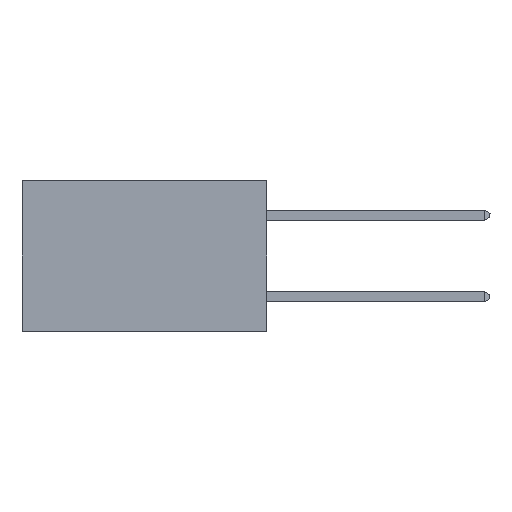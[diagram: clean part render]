
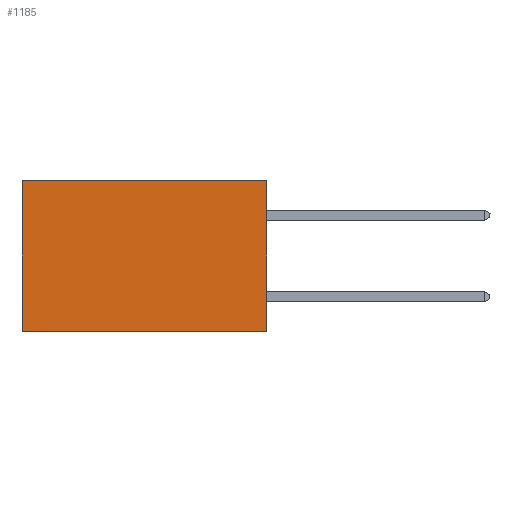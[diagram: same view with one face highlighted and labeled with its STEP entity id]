
A CAD part, left-side view. The second image highlights one B-rep face of the part: STEP entity #1185.
In plain terms, the highlighted planar face has unit normal (-1, 0, 0).
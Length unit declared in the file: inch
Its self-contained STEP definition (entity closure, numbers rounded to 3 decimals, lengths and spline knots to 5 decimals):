
#76 = VECTOR ( 'NONE', #9339, 39.37008 ) ;
#114 = LINE ( 'NONE', #5655, #15353 ) ;
#429 = CARTESIAN_POINT ( 'NONE',  ( 0.2875, 0., 0. ) ) ;
#536 = LINE ( 'NONE', #7866, #76 ) ;
#741 = ORIENTED_EDGE ( 'NONE', *, *, #16037, .F. ) ;
#1185 = ADVANCED_FACE ( 'NONE', ( #12758 ), #17254, .F. ) ;
#1189 = DIRECTION ( 'NONE',  ( 0., 0., -1. ) ) ;
#1426 = EDGE_LOOP ( 'NONE', ( #10645, #2452, #741, #5176 ) ) ;
#1536 = VERTEX_POINT ( 'NONE', #9140 ) ;
#2118 = AXIS2_PLACEMENT_3D ( 'NONE', #15785, #18692, #9932 ) ;
#2452 = ORIENTED_EDGE ( 'NONE', *, *, #13496, .F. ) ;
#3584 = VERTEX_POINT ( 'NONE', #5094 ) ;
#5094 = CARTESIAN_POINT ( 'NONE',  ( 0.2875, 0.6, 0. ) ) ;
#5176 = ORIENTED_EDGE ( 'NONE', *, *, #14701, .T. ) ;
#5655 = CARTESIAN_POINT ( 'NONE',  ( 0.2875, 0., 0. ) ) ;
#6146 = VERTEX_POINT ( 'NONE', #429 ) ;
#7008 = CARTESIAN_POINT ( 'NONE',  ( 0.2875, 0., -0.37 ) ) ;
#7833 = VECTOR ( 'NONE', #1189, 39.37008 ) ;
#7866 = CARTESIAN_POINT ( 'NONE',  ( 0.2875, 0.6, 0. ) ) ;
#8899 = EDGE_CURVE ( 'NONE', #3584, #1536, #536, .T. ) ;
#9140 = CARTESIAN_POINT ( 'NONE',  ( 0.2875, 0.6, -0.37 ) ) ;
#9339 = DIRECTION ( 'NONE',  ( 0., 0., -1. ) ) ;
#9932 = DIRECTION ( 'NONE',  ( 0., 0., -1. ) ) ;
#10038 = CARTESIAN_POINT ( 'NONE',  ( 0.2875, 0., 0. ) ) ;
#10645 = ORIENTED_EDGE ( 'NONE', *, *, #8899, .T. ) ;
#12364 = VECTOR ( 'NONE', #18894, 39.37008 ) ;
#12758 = FACE_OUTER_BOUND ( 'NONE', #1426, .T. ) ;
#12999 = CARTESIAN_POINT ( 'NONE',  ( 0.2875, 0., -0.37 ) ) ;
#13496 = EDGE_CURVE ( 'NONE', #18289, #1536, #17198, .T. ) ;
#14453 = DIRECTION ( 'NONE',  ( 0., 1., 0. ) ) ;
#14701 = EDGE_CURVE ( 'NONE', #6146, #3584, #114, .T. ) ;
#15207 = LINE ( 'NONE', #10038, #7833 ) ;
#15353 = VECTOR ( 'NONE', #14453, 39.37008 ) ;
#15785 = CARTESIAN_POINT ( 'NONE',  ( 0.2875, 0., 0. ) ) ;
#16037 = EDGE_CURVE ( 'NONE', #6146, #18289, #15207, .T. ) ;
#17198 = LINE ( 'NONE', #12999, #12364 ) ;
#17254 = PLANE ( 'NONE',  #2118 ) ;
#18289 = VERTEX_POINT ( 'NONE', #7008 ) ;
#18692 = DIRECTION ( 'NONE',  ( 1., 0., 0. ) ) ;
#18894 = DIRECTION ( 'NONE',  ( 0., 1., 0. ) ) ;
